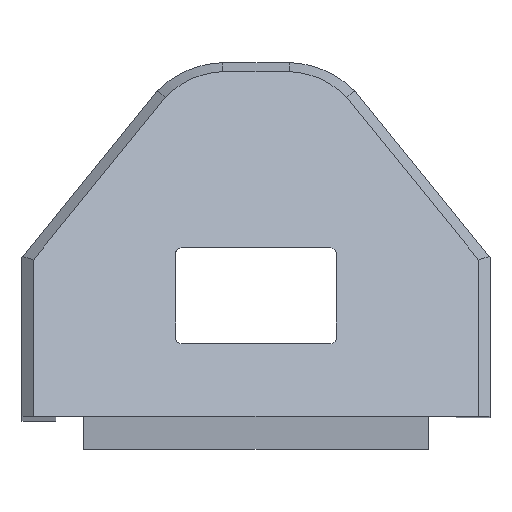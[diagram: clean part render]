
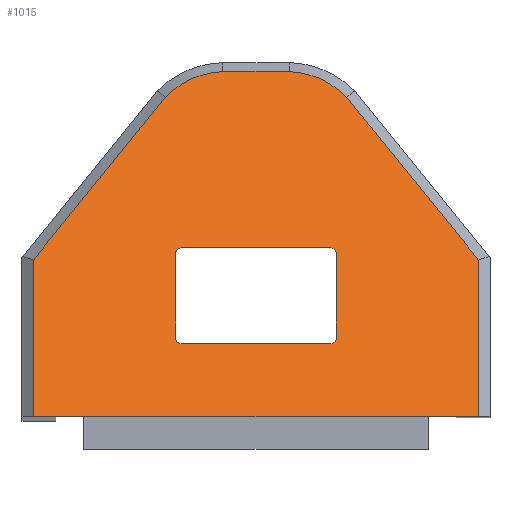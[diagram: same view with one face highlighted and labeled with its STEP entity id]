
A CAD part, top view. The second image highlights one B-rep face of the part: STEP entity #1015.
In plain terms, the highlighted planar face has unit normal (0, 0.603, 0.798).
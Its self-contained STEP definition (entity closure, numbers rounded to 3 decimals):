
#21=B_SPLINE_CURVE_WITH_KNOTS('',3,(#1586,#1587,#1588,#1589,#1590),
 .UNSPECIFIED.,.F.,.F.,(4,1,4),(-3.112,-2.672,-2.338),
 .UNSPECIFIED.);
#22=B_SPLINE_CURVE_WITH_KNOTS('',3,(#1594,#1595,#1596,#1597,#1598),
 .UNSPECIFIED.,.F.,.F.,(4,1,4),(2.338,2.783,3.112),
 .UNSPECIFIED.);
#37=FACE_BOUND('',#170,.T.);
#71=PLANE('',#1110);
#112=FACE_OUTER_BOUND('',#169,.T.);
#169=EDGE_LOOP('',(#775,#776,#777,#778,#779,#780,#781,#782,#783,#784));
#170=EDGE_LOOP('',(#785,#786,#787,#788,#789,#790,#791,#792));
#211=LINE('',#1463,#309);
#214=LINE('',#1475,#312);
#218=LINE('',#1487,#316);
#221=LINE('',#1495,#319);
#247=LINE('',#1573,#345);
#250=LINE('',#1579,#348);
#251=LINE('',#1582,#349);
#252=LINE('',#1584,#350);
#253=LINE('',#1592,#351);
#254=LINE('',#1600,#352);
#255=LINE('',#1602,#353);
#256=LINE('',#1603,#354);
#309=VECTOR('',#1178,10.);
#312=VECTOR('',#1189,10.);
#316=VECTOR('',#1201,10.);
#319=VECTOR('',#1212,10.);
#345=VECTOR('',#1280,10.);
#348=VECTOR('',#1285,10.);
#349=VECTOR('',#1288,10.);
#350=VECTOR('',#1289,10.);
#351=VECTOR('',#1290,10.);
#352=VECTOR('',#1291,10.);
#353=VECTOR('',#1292,10.);
#354=VECTOR('',#1293,10.);
#404=ELLIPSE('',#1074,0.626,0.5);
#405=ELLIPSE('',#1077,0.626,0.5);
#407=ELLIPSE('',#1081,0.626,0.5);
#410=ELLIPSE('',#1086,0.626,0.5);
#425=VERTEX_POINT('',#1453);
#426=VERTEX_POINT('',#1455);
#428=VERTEX_POINT('',#1461);
#429=VERTEX_POINT('',#1465);
#430=VERTEX_POINT('',#1466);
#433=VERTEX_POINT('',#1474);
#435=VERTEX_POINT('',#1480);
#437=VERTEX_POINT('',#1486);
#441=VERTEX_POINT('',#1501);
#446=VERTEX_POINT('',#1512);
#468=VERTEX_POINT('',#1577);
#469=VERTEX_POINT('',#1581);
#470=VERTEX_POINT('',#1583);
#471=VERTEX_POINT('',#1585);
#472=VERTEX_POINT('',#1591);
#473=VERTEX_POINT('',#1593);
#474=VERTEX_POINT('',#1599);
#475=VERTEX_POINT('',#1601);
#524=EDGE_CURVE('',#425,#426,#404,.T.);
#528=EDGE_CURVE('',#425,#428,#211,.T.);
#529=EDGE_CURVE('',#429,#430,#405,.T.);
#533=EDGE_CURVE('',#433,#430,#214,.T.);
#536=EDGE_CURVE('',#433,#435,#407,.T.);
#539=EDGE_CURVE('',#437,#435,#218,.T.);
#543=EDGE_CURVE('',#437,#428,#410,.T.);
#544=EDGE_CURVE('',#429,#426,#221,.T.);
#582=EDGE_CURVE('',#446,#441,#247,.T.);
#585=EDGE_CURVE('',#468,#446,#250,.T.);
#586=EDGE_CURVE('',#469,#468,#251,.T.);
#587=EDGE_CURVE('',#470,#469,#252,.T.);
#588=EDGE_CURVE('',#471,#470,#21,.T.);
#589=EDGE_CURVE('',#472,#471,#253,.T.);
#590=EDGE_CURVE('',#473,#472,#22,.T.);
#591=EDGE_CURVE('',#474,#473,#254,.T.);
#592=EDGE_CURVE('',#475,#474,#255,.T.);
#593=EDGE_CURVE('',#441,#475,#256,.T.);
#775=ORIENTED_EDGE('',*,*,#586,.F.);
#776=ORIENTED_EDGE('',*,*,#587,.F.);
#777=ORIENTED_EDGE('',*,*,#588,.F.);
#778=ORIENTED_EDGE('',*,*,#589,.F.);
#779=ORIENTED_EDGE('',*,*,#590,.F.);
#780=ORIENTED_EDGE('',*,*,#591,.F.);
#781=ORIENTED_EDGE('',*,*,#592,.F.);
#782=ORIENTED_EDGE('',*,*,#593,.F.);
#783=ORIENTED_EDGE('',*,*,#582,.F.);
#784=ORIENTED_EDGE('',*,*,#585,.F.);
#785=ORIENTED_EDGE('',*,*,#544,.T.);
#786=ORIENTED_EDGE('',*,*,#524,.F.);
#787=ORIENTED_EDGE('',*,*,#528,.T.);
#788=ORIENTED_EDGE('',*,*,#543,.F.);
#789=ORIENTED_EDGE('',*,*,#539,.T.);
#790=ORIENTED_EDGE('',*,*,#536,.F.);
#791=ORIENTED_EDGE('',*,*,#533,.T.);
#792=ORIENTED_EDGE('',*,*,#529,.F.);
#1015=ADVANCED_FACE('',(#112,#37),#71,.T.);
#1074=AXIS2_PLACEMENT_3D('',#1456,#1171,#1172);
#1077=AXIS2_PLACEMENT_3D('',#1467,#1181,#1182);
#1081=AXIS2_PLACEMENT_3D('',#1481,#1194,#1195);
#1086=AXIS2_PLACEMENT_3D('',#1493,#1208,#1209);
#1110=AXIS2_PLACEMENT_3D('',#1580,#1286,#1287);
#1171=DIRECTION('center_axis',(0.,0.602,0.798));
#1172=DIRECTION('ref_axis',(0.,0.798,-0.602));
#1178=DIRECTION('',(0.,-0.798,0.602));
#1181=DIRECTION('center_axis',(0.,0.602,0.798));
#1182=DIRECTION('ref_axis',(0.,0.798,-0.602));
#1189=DIRECTION('',(0.,0.798,-0.602));
#1194=DIRECTION('center_axis',(0.,0.602,0.798));
#1195=DIRECTION('ref_axis',(0.,-0.798,0.602));
#1201=DIRECTION('',(-1.,0.,0.));
#1208=DIRECTION('center_axis',(0.,0.602,0.798));
#1209=DIRECTION('ref_axis',(0.,-0.798,0.602));
#1212=DIRECTION('',(1.,0.,0.));
#1280=DIRECTION('',(-1.,0.,0.));
#1285=DIRECTION('',(-1.,0.,0.));
#1286=DIRECTION('center_axis',(0.,0.602,0.798));
#1287=DIRECTION('ref_axis',(1.,0.,0.));
#1288=DIRECTION('',(0.,-0.798,0.602));
#1289=DIRECTION('',(0.543,-0.67,0.506));
#1290=DIRECTION('',(1.,0.,0.));
#1291=DIRECTION('',(0.543,0.67,-0.506));
#1292=DIRECTION('',(0.,0.798,-0.602));
#1293=DIRECTION('',(-1.,0.,0.));
#1453=CARTESIAN_POINT('',(7.119,14.144,246.885));
#1455=CARTESIAN_POINT('',(6.619,14.644,246.507));
#1456=CARTESIAN_POINT('Origin',(6.619,14.144,246.885));
#1461=CARTESIAN_POINT('',(7.119,6.644,252.546));
#1463=CARTESIAN_POINT('',(7.119,68.652,205.737));
#1465=CARTESIAN_POINT('',(-6.619,14.644,246.507));
#1466=CARTESIAN_POINT('',(-7.119,14.144,246.885));
#1467=CARTESIAN_POINT('Origin',(-6.619,14.144,246.885));
#1474=CARTESIAN_POINT('',(-7.119,6.644,252.546));
#1475=CARTESIAN_POINT('',(-7.119,71.041,203.934));
#1480=CARTESIAN_POINT('',(-6.619,6.144,252.924));
#1481=CARTESIAN_POINT('Origin',(-6.619,6.644,252.546));
#1486=CARTESIAN_POINT('',(6.619,6.144,252.924));
#1487=CARTESIAN_POINT('',(-8.738,6.144,252.924));
#1493=CARTESIAN_POINT('Origin',(6.619,6.644,252.546));
#1495=CARTESIAN_POINT('',(-1.619,14.644,246.507));
#1501=CARTESIAN_POINT('',(-15.24,-0.294,257.784));
#1512=CARTESIAN_POINT('',(15.24,-0.294,257.784));
#1573=CARTESIAN_POINT('',(-14.045,-0.294,257.784));
#1577=CARTESIAN_POINT('',(19.715,-0.294,257.784));
#1579=CARTESIAN_POINT('',(-14.045,-0.294,257.784));
#1580=CARTESIAN_POINT('Origin',(-10.358,16.518,245.093));
#1581=CARTESIAN_POINT('',(19.715,13.564,247.323));
#1582=CARTESIAN_POINT('',(19.715,68.818,205.612));
#1583=CARTESIAN_POINT('',(8.037,27.981,236.439));
#1584=CARTESIAN_POINT('',(-19.426,61.884,210.846));
#1585=CARTESIAN_POINT('',(2.934,30.262,234.717));
#1586=CARTESIAN_POINT('Ctrl Pts',(2.934,30.262,234.717));
#1587=CARTESIAN_POINT('Ctrl Pts',(3.995,30.23,234.741));
#1588=CARTESIAN_POINT('Ctrl Pts',(5.856,29.761,235.096));
#1589=CARTESIAN_POINT('Ctrl Pts',(7.446,28.592,235.978));
#1590=CARTESIAN_POINT('Ctrl Pts',(8.037,27.981,236.439));
#1591=CARTESIAN_POINT('',(-2.934,30.262,234.717));
#1592=CARTESIAN_POINT('',(-3.703,30.262,234.717));
#1593=CARTESIAN_POINT('',(-8.037,27.981,236.439));
#1594=CARTESIAN_POINT('Ctrl Pts',(-8.037,27.981,236.439));
#1595=CARTESIAN_POINT('Ctrl Pts',(-7.25,28.796,235.824));
#1596=CARTESIAN_POINT('Ctrl Pts',(-5.588,29.877,235.008));
#1597=CARTESIAN_POINT('Ctrl Pts',(-3.726,30.238,234.735));
#1598=CARTESIAN_POINT('Ctrl Pts',(-2.934,30.262,234.717));
#1599=CARTESIAN_POINT('',(-19.715,13.564,247.323));
#1600=CARTESIAN_POINT('',(16.373,58.115,213.692));
#1601=CARTESIAN_POINT('',(-19.715,-0.294,257.784));
#1602=CARTESIAN_POINT('',(-19.715,68.818,205.612));
#1603=CARTESIAN_POINT('',(-14.045,-0.294,257.784));
